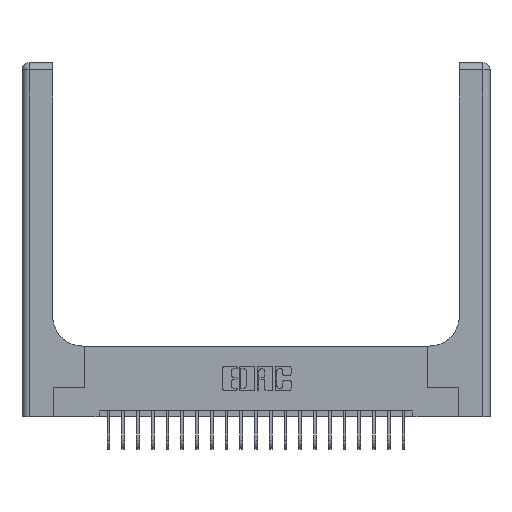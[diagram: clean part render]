
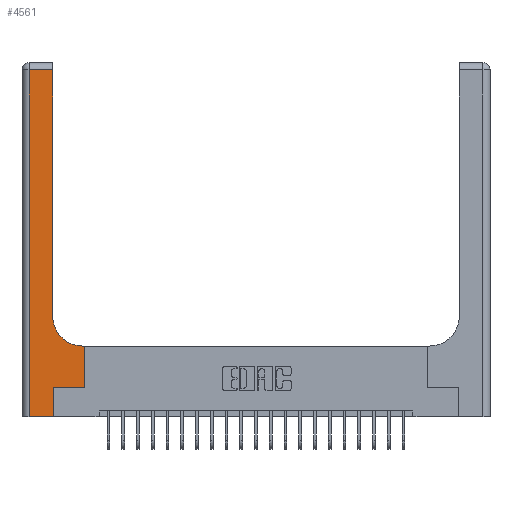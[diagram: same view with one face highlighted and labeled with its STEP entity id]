
A CAD part, top view. The second image highlights one B-rep face of the part: STEP entity #4561.
In plain terms, the highlighted planar face has unit normal (0, 0, 1).
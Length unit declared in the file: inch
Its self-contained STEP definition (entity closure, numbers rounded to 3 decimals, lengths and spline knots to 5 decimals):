
#441 = VERTEX_POINT ( 'NONE', #10721 ) ;
#516 = VERTEX_POINT ( 'NONE', #13047 ) ;
#558 = EDGE_LOOP ( 'NONE', ( #4467, #22206, #13054, #14593, #17659, #11807, #7142, #14061, #6964 ) ) ;
#745 = LINE ( 'NONE', #13219, #19510 ) ;
#951 = EDGE_CURVE ( 'NONE', #10789, #9098, #745, .T. ) ;
#1002 = LINE ( 'NONE', #14199, #23301 ) ;
#1121 = DIRECTION ( 'NONE',  ( 0., 1., 0. ) ) ;
#1197 = DIRECTION ( 'NONE',  ( 1., 0., 0. ) ) ;
#2708 = CARTESIAN_POINT ( 'NONE',  ( 0.265, 0., 0.37 ) ) ;
#3205 = LINE ( 'NONE', #8751, #13266 ) ;
#3455 = DIRECTION ( 'NONE',  ( 0., 1., 0. ) ) ;
#3857 = EDGE_CURVE ( 'NONE', #6702, #7211, #3924, .T. ) ;
#3924 = LINE ( 'NONE', #13146, #9196 ) ;
#4390 = DIRECTION ( 'NONE',  ( -1., 0., 0. ) ) ;
#4411 = VECTOR ( 'NONE', #1121, 39.37008 ) ;
#4467 = ORIENTED_EDGE ( 'NONE', *, *, #11997, .T. ) ;
#4561 = ADVANCED_FACE ( 'NONE', ( #13953 ), #12127, .F. ) ;
#5819 = DIRECTION ( 'NONE',  ( -1., 0., 0. ) ) ;
#5929 = LINE ( 'NONE', #17336, #18547 ) ;
#5977 = EDGE_CURVE ( 'NONE', #22768, #6702, #5929, .T. ) ;
#6540 = CARTESIAN_POINT ( 'NONE',  ( 0.265, 0.25, 0.37 ) ) ;
#6702 = VERTEX_POINT ( 'NONE', #9429 ) ;
#6799 = DIRECTION ( 'NONE',  ( 1., 0., 0. ) ) ;
#6964 = ORIENTED_EDGE ( 'NONE', *, *, #19532, .T. ) ;
#7142 = ORIENTED_EDGE ( 'NONE', *, *, #3857, .T. ) ;
#7211 = VERTEX_POINT ( 'NONE', #8730 ) ;
#7311 = VERTEX_POINT ( 'NONE', #18579 ) ;
#7428 = EDGE_CURVE ( 'NONE', #7211, #441, #8022, .T. ) ;
#8022 = LINE ( 'NONE', #15550, #21268 ) ;
#8038 = AXIS2_PLACEMENT_3D ( 'NONE', #12007, #19397, #17602 ) ;
#8730 = CARTESIAN_POINT ( 'NONE',  ( 0.528, 0.6, 0.37 ) ) ;
#8751 = CARTESIAN_POINT ( 'NONE',  ( 0.26, 3., 0.37 ) ) ;
#9098 = VERTEX_POINT ( 'NONE', #13703 ) ;
#9196 = VECTOR ( 'NONE', #3455, 39.37008 ) ;
#9429 = CARTESIAN_POINT ( 'NONE',  ( 0.528, 0.25, 0.37 ) ) ;
#9761 = AXIS2_PLACEMENT_3D ( 'NONE', #10381, #17701, #1197 ) ;
#10381 = CARTESIAN_POINT ( 'NONE',  ( 0.51, 0.85, 0.37 ) ) ;
#10721 = CARTESIAN_POINT ( 'NONE',  ( 0.51, 0.6, 0.37 ) ) ;
#10789 = VERTEX_POINT ( 'NONE', #19575 ) ;
#10950 = DIRECTION ( 'NONE',  ( 0., 1., 0. ) ) ;
#11080 = CARTESIAN_POINT ( 'NONE',  ( 0.06, 0., 0.37 ) ) ;
#11499 = DIRECTION ( 'NONE',  ( 1., 0., 0. ) ) ;
#11806 = CARTESIAN_POINT ( 'NONE',  ( 0.06, 3., 0.37 ) ) ;
#11807 = ORIENTED_EDGE ( 'NONE', *, *, #5977, .T. ) ;
#11909 = LINE ( 'NONE', #2708, #4411 ) ;
#11997 = EDGE_CURVE ( 'NONE', #516, #10789, #3205, .T. ) ;
#12007 = CARTESIAN_POINT ( 'NONE',  ( 0., 3., 0.37 ) ) ;
#12127 = PLANE ( 'NONE',  #8038 ) ;
#13047 = CARTESIAN_POINT ( 'NONE',  ( 0.26, 0.85, 0.37 ) ) ;
#13054 = ORIENTED_EDGE ( 'NONE', *, *, #23674, .T. ) ;
#13146 = CARTESIAN_POINT ( 'NONE',  ( 0.528, 0.25, 0.37 ) ) ;
#13219 = CARTESIAN_POINT ( 'NONE',  ( 0., 2.94, 0.37 ) ) ;
#13266 = VECTOR ( 'NONE', #10950, 39.37008 ) ;
#13269 = CIRCLE ( 'NONE', #9761, 0.25 ) ;
#13637 = LINE ( 'NONE', #11806, #20324 ) ;
#13703 = CARTESIAN_POINT ( 'NONE',  ( 0.06, 2.94, 0.37 ) ) ;
#13953 = FACE_OUTER_BOUND ( 'NONE', #558, .T. ) ;
#14061 = ORIENTED_EDGE ( 'NONE', *, *, #7428, .T. ) ;
#14199 = CARTESIAN_POINT ( 'NONE',  ( 0., 0., 0.37 ) ) ;
#14593 = ORIENTED_EDGE ( 'NONE', *, *, #17999, .T. ) ;
#15550 = CARTESIAN_POINT ( 'NONE',  ( 0.26, 0.6, 0.37 ) ) ;
#17336 = CARTESIAN_POINT ( 'NONE',  ( 0.265, 0.25, 0.37 ) ) ;
#17602 = DIRECTION ( 'NONE',  ( -1., 0., 0. ) ) ;
#17659 = ORIENTED_EDGE ( 'NONE', *, *, #21998, .T. ) ;
#17701 = DIRECTION ( 'NONE',  ( 0., 0., -1. ) ) ;
#17999 = EDGE_CURVE ( 'NONE', #19971, #7311, #1002, .T. ) ;
#18547 = VECTOR ( 'NONE', #11499, 39.37008 ) ;
#18579 = CARTESIAN_POINT ( 'NONE',  ( 0.265, 0., 0.37 ) ) ;
#19202 = DIRECTION ( 'NONE',  ( 0., -1., 0. ) ) ;
#19397 = DIRECTION ( 'NONE',  ( 0., 0., -1. ) ) ;
#19510 = VECTOR ( 'NONE', #5819, 39.37008 ) ;
#19532 = EDGE_CURVE ( 'NONE', #441, #516, #13269, .T. ) ;
#19575 = CARTESIAN_POINT ( 'NONE',  ( 0.26, 2.94, 0.37 ) ) ;
#19971 = VERTEX_POINT ( 'NONE', #11080 ) ;
#20324 = VECTOR ( 'NONE', #19202, 39.37008 ) ;
#21268 = VECTOR ( 'NONE', #4390, 39.37008 ) ;
#21998 = EDGE_CURVE ( 'NONE', #7311, #22768, #11909, .T. ) ;
#22206 = ORIENTED_EDGE ( 'NONE', *, *, #951, .T. ) ;
#22768 = VERTEX_POINT ( 'NONE', #6540 ) ;
#23301 = VECTOR ( 'NONE', #6799, 39.37008 ) ;
#23674 = EDGE_CURVE ( 'NONE', #9098, #19971, #13637, .T. ) ;
